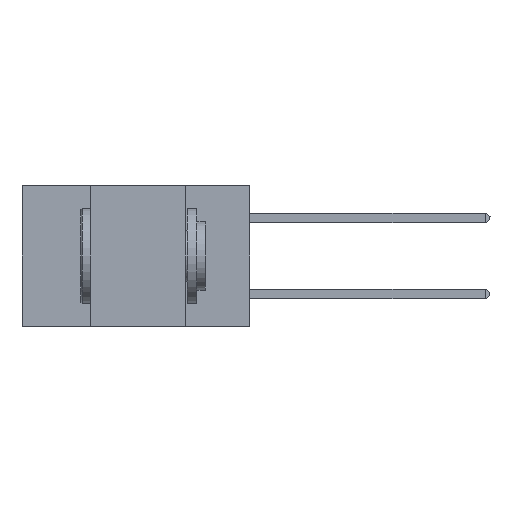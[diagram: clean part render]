
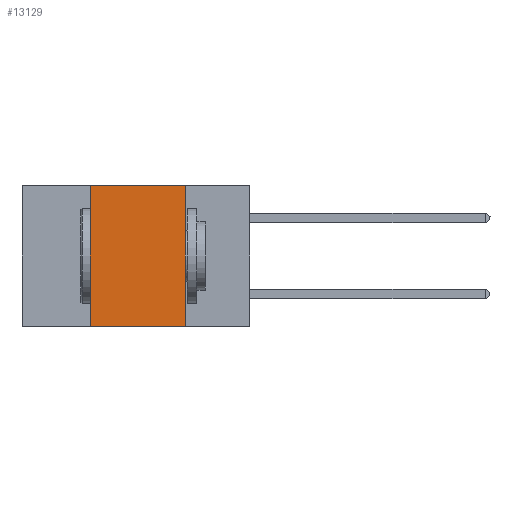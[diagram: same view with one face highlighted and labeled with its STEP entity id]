
A CAD part, left-side view. The second image highlights one B-rep face of the part: STEP entity #13129.
In plain terms, the highlighted planar face has unit normal (-1, 0, 0).
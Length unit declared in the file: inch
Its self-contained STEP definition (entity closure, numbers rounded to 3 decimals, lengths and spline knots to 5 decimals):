
#136 = ORIENTED_EDGE ( 'NONE', *, *, #3778, .F. ) ;
#3778 = EDGE_CURVE ( 'NONE', #31647, #10884, #11634, .T. ) ;
#4294 = FACE_OUTER_BOUND ( 'NONE', #20944, .T. ) ;
#4839 = LINE ( 'NONE', #15311, #10752 ) ;
#4939 = VECTOR ( 'NONE', #10417, 39.37008 ) ;
#4997 = VECTOR ( 'NONE', #29740, 39.37008 ) ;
#6332 = VERTEX_POINT ( 'NONE', #20046 ) ;
#6585 = CARTESIAN_POINT ( 'NONE',  ( 0., 0.6, -0.37 ) ) ;
#6990 = EDGE_CURVE ( 'NONE', #6332, #31647, #18365, .T. ) ;
#9320 = ORIENTED_EDGE ( 'NONE', *, *, #31206, .F. ) ;
#9874 = CARTESIAN_POINT ( 'NONE',  ( 0., 0.6, 0. ) ) ;
#10100 = ORIENTED_EDGE ( 'NONE', *, *, #17908, .T. ) ;
#10207 = CARTESIAN_POINT ( 'NONE',  ( 0., 0.42, -0.37 ) ) ;
#10417 = DIRECTION ( 'NONE',  ( 0., 0., -1. ) ) ;
#10752 = VECTOR ( 'NONE', #17733, 39.37008 ) ;
#10884 = VERTEX_POINT ( 'NONE', #18225 ) ;
#11634 = LINE ( 'NONE', #30349, #4939 ) ;
#13129 = ADVANCED_FACE ( 'NONE', ( #4294 ), #14924, .F. ) ;
#13604 = DIRECTION ( 'NONE',  ( 0., -1., 0. ) ) ;
#14241 = VECTOR ( 'NONE', #13604, 39.37008 ) ;
#14924 = PLANE ( 'NONE',  #23207 ) ;
#15311 = CARTESIAN_POINT ( 'NONE',  ( 0., 0.42, 0. ) ) ;
#16609 = VERTEX_POINT ( 'NONE', #10207 ) ;
#17456 = DIRECTION ( 'NONE',  ( 0., 0., -1. ) ) ;
#17733 = DIRECTION ( 'NONE',  ( 0., 0., 1. ) ) ;
#17908 = EDGE_CURVE ( 'NONE', #16609, #10884, #20933, .T. ) ;
#18225 = CARTESIAN_POINT ( 'NONE',  ( 0., 0.17, -0.37 ) ) ;
#18365 = LINE ( 'NONE', #19900, #4997 ) ;
#19482 = CARTESIAN_POINT ( 'NONE',  ( 0., 0.17, 0. ) ) ;
#19900 = CARTESIAN_POINT ( 'NONE',  ( 0., 0.6, 0. ) ) ;
#20046 = CARTESIAN_POINT ( 'NONE',  ( 0., 0.42, 0. ) ) ;
#20933 = LINE ( 'NONE', #6585, #14241 ) ;
#20944 = EDGE_LOOP ( 'NONE', ( #136, #26927, #9320, #10100 ) ) ;
#23207 = AXIS2_PLACEMENT_3D ( 'NONE', #9874, #32304, #17456 ) ;
#26927 = ORIENTED_EDGE ( 'NONE', *, *, #6990, .F. ) ;
#29740 = DIRECTION ( 'NONE',  ( 0., -1., 0. ) ) ;
#30349 = CARTESIAN_POINT ( 'NONE',  ( 0., 0.17, 0. ) ) ;
#31206 = EDGE_CURVE ( 'NONE', #16609, #6332, #4839, .T. ) ;
#31647 = VERTEX_POINT ( 'NONE', #19482 ) ;
#32304 = DIRECTION ( 'NONE',  ( 1., 0., 0. ) ) ;
